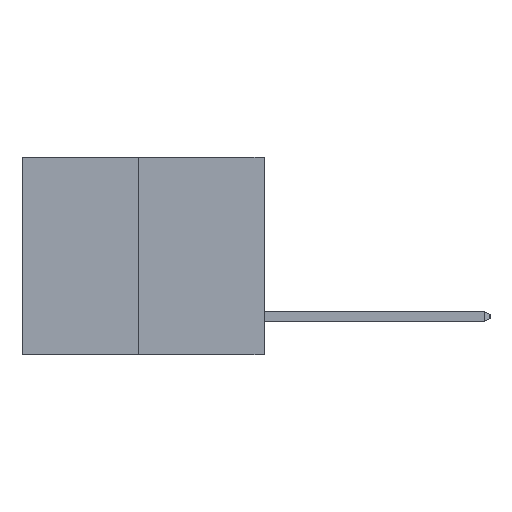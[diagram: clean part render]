
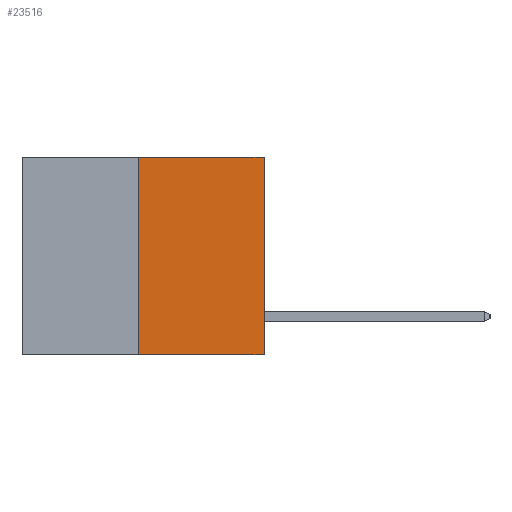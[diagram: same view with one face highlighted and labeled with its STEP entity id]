
A CAD part, left-side view. The second image highlights one B-rep face of the part: STEP entity #23516.
In plain terms, the highlighted planar face has unit normal (-1, 0, 0).
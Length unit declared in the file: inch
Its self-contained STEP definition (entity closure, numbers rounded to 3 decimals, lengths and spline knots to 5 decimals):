
#326 = VERTEX_POINT ( 'NONE', #23198 ) ;
#567 = CARTESIAN_POINT ( 'NONE',  ( 0., 0., 0. ) ) ;
#1430 = EDGE_CURVE ( 'NONE', #3413, #8449, #19328, .T. ) ;
#2294 = DIRECTION ( 'NONE',  ( 0., 0., 1. ) ) ;
#3062 = EDGE_LOOP ( 'NONE', ( #11702, #8467, #6247, #22166 ) ) ;
#3413 = VERTEX_POINT ( 'NONE', #20429 ) ;
#3896 = LINE ( 'NONE', #9907, #23427 ) ;
#4226 = AXIS2_PLACEMENT_3D ( 'NONE', #16211, #6808, #20181 ) ;
#4258 = LINE ( 'NONE', #567, #22073 ) ;
#5041 = VECTOR ( 'NONE', #22509, 39.37008 ) ;
#5276 = EDGE_CURVE ( 'NONE', #3413, #326, #3896, .T. ) ;
#5302 = DIRECTION ( 'NONE',  ( 0., 0., 1. ) ) ;
#5941 = VERTEX_POINT ( 'NONE', #20511 ) ;
#6247 = ORIENTED_EDGE ( 'NONE', *, *, #21829, .T. ) ;
#6808 = DIRECTION ( 'NONE',  ( 1., 0., 0. ) ) ;
#7279 = CARTESIAN_POINT ( 'NONE',  ( 0., 0.6, -0.49 ) ) ;
#7683 = DIRECTION ( 'NONE',  ( 0., -1., 0. ) ) ;
#8449 = VERTEX_POINT ( 'NONE', #19360 ) ;
#8467 = ORIENTED_EDGE ( 'NONE', *, *, #1430, .T. ) ;
#9069 = EDGE_CURVE ( 'NONE', #326, #5941, #20188, .T. ) ;
#9907 = CARTESIAN_POINT ( 'NONE',  ( 0., 0.312, -0.49 ) ) ;
#11702 = ORIENTED_EDGE ( 'NONE', *, *, #5276, .F. ) ;
#12551 = PLANE ( 'NONE',  #4226 ) ;
#12874 = FACE_OUTER_BOUND ( 'NONE', #3062, .T. ) ;
#15140 = VECTOR ( 'NONE', #7683, 39.37008 ) ;
#15402 = CARTESIAN_POINT ( 'NONE',  ( 0., 0.6, 0. ) ) ;
#16211 = CARTESIAN_POINT ( 'NONE',  ( 0., 0.6, 0. ) ) ;
#19328 = LINE ( 'NONE', #7279, #5041 ) ;
#19360 = CARTESIAN_POINT ( 'NONE',  ( 0., 0., -0.49 ) ) ;
#20181 = DIRECTION ( 'NONE',  ( 0., 0., -1. ) ) ;
#20188 = LINE ( 'NONE', #15402, #15140 ) ;
#20429 = CARTESIAN_POINT ( 'NONE',  ( 0., 0.312, -0.49 ) ) ;
#20511 = CARTESIAN_POINT ( 'NONE',  ( 0., 0., 0. ) ) ;
#21829 = EDGE_CURVE ( 'NONE', #8449, #5941, #4258, .T. ) ;
#22073 = VECTOR ( 'NONE', #2294, 39.37008 ) ;
#22166 = ORIENTED_EDGE ( 'NONE', *, *, #9069, .F. ) ;
#22509 = DIRECTION ( 'NONE',  ( 0., -1., 0. ) ) ;
#23198 = CARTESIAN_POINT ( 'NONE',  ( 0., 0.312, 0. ) ) ;
#23427 = VECTOR ( 'NONE', #5302, 39.37008 ) ;
#23516 = ADVANCED_FACE ( 'NONE', ( #12874 ), #12551, .F. ) ;
